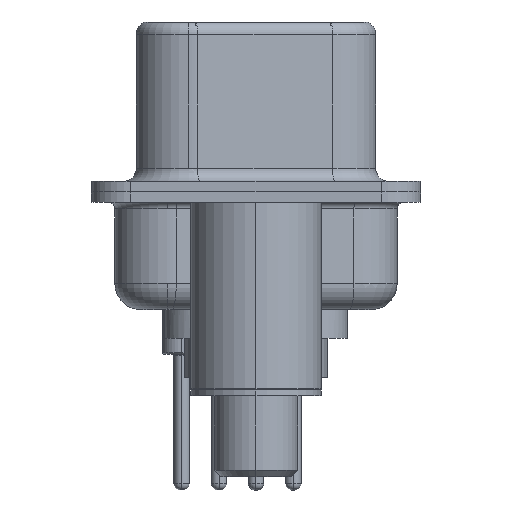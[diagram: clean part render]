
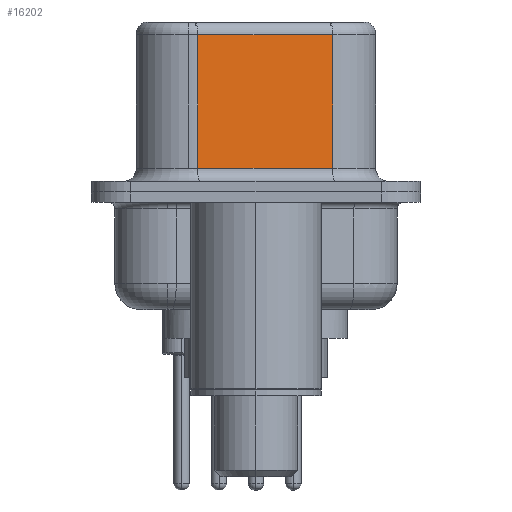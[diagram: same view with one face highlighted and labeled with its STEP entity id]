
A CAD part, left-side view. The second image highlights one B-rep face of the part: STEP entity #16202.
In plain terms, the highlighted planar face has unit normal (-0.985, -0.174, 0).
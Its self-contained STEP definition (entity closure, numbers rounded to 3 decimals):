
#915 = FACE_OUTER_BOUND ( 'NONE', #18843, .T. ) ;
#982 = VECTOR ( 'NONE', #21263, 1000. ) ;
#1188 = VERTEX_POINT ( 'NONE', #1610 ) ;
#1610 = CARTESIAN_POINT ( 'NONE',  ( 3.67, 2.233, 0.9 ) ) ;
#1854 = EDGE_CURVE ( 'NONE', #1188, #2265, #3235, .T. ) ;
#2265 = VERTEX_POINT ( 'NONE', #18151 ) ;
#2685 = ORIENTED_EDGE ( 'NONE', *, *, #4531, .T. ) ;
#3235 = LINE ( 'NONE', #12200, #21743 ) ;
#4126 = CARTESIAN_POINT ( 'NONE',  ( 3.67, 2.233, 6.52 ) ) ;
#4531 = EDGE_CURVE ( 'NONE', #7979, #5069, #9076, .T. ) ;
#4761 = ORIENTED_EDGE ( 'NONE', *, *, #21733, .F. ) ;
#5069 = VERTEX_POINT ( 'NONE', #20570 ) ;
#7610 = CARTESIAN_POINT ( 'NONE',  ( 4.58, -2.927, 6.02 ) ) ;
#7979 = VERTEX_POINT ( 'NONE', #19213 ) ;
#8388 = ORIENTED_EDGE ( 'NONE', *, *, #17738, .T. ) ;
#8574 = DIRECTION ( 'NONE',  ( -0.174, 0.985, 0. ) ) ;
#9076 = LINE ( 'NONE', #7610, #18616 ) ;
#10615 = CARTESIAN_POINT ( 'NONE',  ( 4.58, -2.927, 6.52 ) ) ;
#10658 = DIRECTION ( 'NONE',  ( 0.985, 0.174, 0. ) ) ;
#10822 = ORIENTED_EDGE ( 'NONE', *, *, #1854, .T. ) ;
#11098 = VECTOR ( 'NONE', #14921, 1000. ) ;
#12200 = CARTESIAN_POINT ( 'NONE',  ( 4.58, -2.927, 0.9 ) ) ;
#12877 = AXIS2_PLACEMENT_3D ( 'NONE', #21302, #10658, #23083 ) ;
#14921 = DIRECTION ( 'NONE',  ( 0., 0., -1. ) ) ;
#16202 = ADVANCED_FACE ( 'NONE', ( #915 ), #17741, .F. ) ;
#17738 = EDGE_CURVE ( 'NONE', #5069, #1188, #21071, .T. ) ;
#17741 = PLANE ( 'NONE',  #12877 ) ;
#18151 = CARTESIAN_POINT ( 'NONE',  ( 4.58, -2.927, 0.9 ) ) ;
#18616 = VECTOR ( 'NONE', #8574, 1000. ) ;
#18843 = EDGE_LOOP ( 'NONE', ( #4761, #2685, #8388, #10822 ) ) ;
#19213 = CARTESIAN_POINT ( 'NONE',  ( 4.58, -2.927, 6.02 ) ) ;
#20128 = LINE ( 'NONE', #10615, #982 ) ;
#20570 = CARTESIAN_POINT ( 'NONE',  ( 3.67, 2.233, 6.02 ) ) ;
#21071 = LINE ( 'NONE', #4126, #11098 ) ;
#21263 = DIRECTION ( 'NONE',  ( 0., 0., -1. ) ) ;
#21302 = CARTESIAN_POINT ( 'NONE',  ( 4.58, -2.927, 6.52 ) ) ;
#21733 = EDGE_CURVE ( 'NONE', #7979, #2265, #20128, .T. ) ;
#21743 = VECTOR ( 'NONE', #22750, 1000. ) ;
#22750 = DIRECTION ( 'NONE',  ( 0.174, -0.985, 0. ) ) ;
#23083 = DIRECTION ( 'NONE',  ( -0.174, 0.985, 0. ) ) ;
